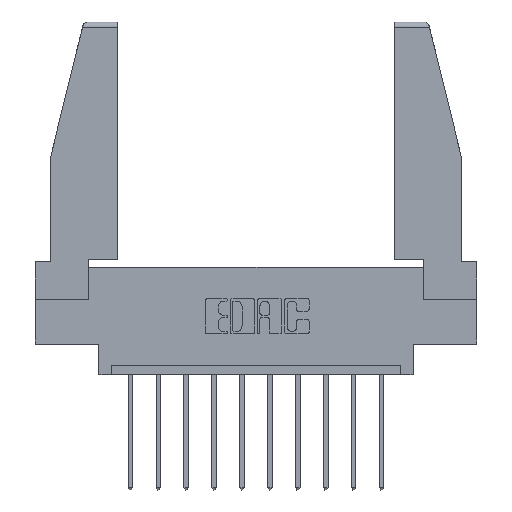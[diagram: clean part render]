
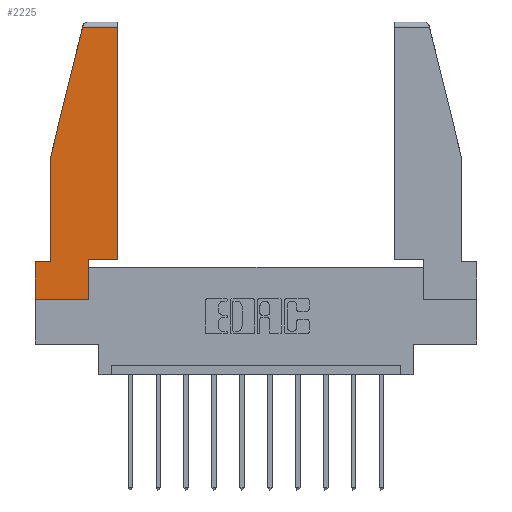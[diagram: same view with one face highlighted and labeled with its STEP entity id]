
A CAD part, top view. The second image highlights one B-rep face of the part: STEP entity #2225.
In plain terms, the highlighted planar face has unit normal (0, 0, 1).
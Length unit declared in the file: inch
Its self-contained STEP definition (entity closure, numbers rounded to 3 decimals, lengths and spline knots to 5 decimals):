
#368 = LINE ( 'NONE', #5618, #10262 ) ;
#378 = VERTEX_POINT ( 'NONE', #9417 ) ;
#496 = LINE ( 'NONE', #4893, #7648 ) ;
#766 = EDGE_CURVE ( 'NONE', #2011, #13104, #2961, .T. ) ;
#790 = CARTESIAN_POINT ( 'NONE',  ( 0.297, 0., 0. ) ) ;
#1010 = LINE ( 'NONE', #7868, #7314 ) ;
#1463 = VERTEX_POINT ( 'NONE', #4275 ) ;
#1689 = CARTESIAN_POINT ( 'NONE',  ( 0., 0., 0. ) ) ;
#1738 = CARTESIAN_POINT ( 'NONE',  ( 0.297, 0.223, 0. ) ) ;
#1741 = VECTOR ( 'NONE', #7328, 39.37008 ) ;
#1757 = CARTESIAN_POINT ( 'NONE',  ( 0., 0., 0. ) ) ;
#1901 = ORIENTED_EDGE ( 'NONE', *, *, #5869, .T. ) ;
#2002 = VERTEX_POINT ( 'NONE', #13920 ) ;
#2011 = VERTEX_POINT ( 'NONE', #790 ) ;
#2225 = ADVANCED_FACE ( 'NONE', ( #13808 ), #8231, .T. ) ;
#2400 = ORIENTED_EDGE ( 'NONE', *, *, #5689, .T. ) ;
#2610 = CARTESIAN_POINT ( 'NONE',  ( 0.2636, 1.52, 0. ) ) ;
#2647 = CARTESIAN_POINT ( 'NONE',  ( 0.271, 1.55, 0. ) ) ;
#2772 = EDGE_LOOP ( 'NONE', ( #13623, #6765, #2400, #9974, #5412, #1901, #4437, #6620, #4137 ) ) ;
#2961 = LINE ( 'NONE', #13052, #10128 ) ;
#3959 = VECTOR ( 'NONE', #10266, 39.37008 ) ;
#4137 = ORIENTED_EDGE ( 'NONE', *, *, #10483, .T. ) ;
#4158 = VECTOR ( 'NONE', #13670, 39.37008 ) ;
#4275 = CARTESIAN_POINT ( 'NONE',  ( 0.086, 0.21, 0. ) ) ;
#4437 = ORIENTED_EDGE ( 'NONE', *, *, #5126, .T. ) ;
#4545 = DIRECTION ( 'NONE',  ( 0., -1., 0. ) ) ;
#4553 = CARTESIAN_POINT ( 'NONE',  ( 0.461, 1.52, 0. ) ) ;
#4643 = LINE ( 'NONE', #7715, #5138 ) ;
#4893 = CARTESIAN_POINT ( 'NONE',  ( 0., 0.21, 0. ) ) ;
#5126 = EDGE_CURVE ( 'NONE', #2002, #2011, #12850, .T. ) ;
#5138 = VECTOR ( 'NONE', #4545, 39.37008 ) ;
#5264 = DIRECTION ( 'NONE',  ( 1., 0., 0. ) ) ;
#5412 = ORIENTED_EDGE ( 'NONE', *, *, #12501, .T. ) ;
#5604 = LINE ( 'NONE', #6216, #11063 ) ;
#5618 = CARTESIAN_POINT ( 'NONE',  ( 0., 1.52, 0. ) ) ;
#5625 = DIRECTION ( 'NONE',  ( 0., -1., 0. ) ) ;
#5689 = EDGE_CURVE ( 'NONE', #11880, #10611, #11294, .T. ) ;
#5869 = EDGE_CURVE ( 'NONE', #378, #2002, #4643, .T. ) ;
#6016 = DIRECTION ( 'NONE',  ( -1., 0., 0. ) ) ;
#6216 = CARTESIAN_POINT ( 'NONE',  ( 0.461, 0.223, 0. ) ) ;
#6609 = DIRECTION ( 'NONE',  ( -1., 0., 0. ) ) ;
#6620 = ORIENTED_EDGE ( 'NONE', *, *, #766, .T. ) ;
#6765 = ORIENTED_EDGE ( 'NONE', *, *, #10817, .T. ) ;
#7008 = LINE ( 'NONE', #13935, #1741 ) ;
#7314 = VECTOR ( 'NONE', #5625, 39.37008 ) ;
#7328 = DIRECTION ( 'NONE',  ( 1., 0., 0. ) ) ;
#7648 = VECTOR ( 'NONE', #6016, 39.37008 ) ;
#7715 = CARTESIAN_POINT ( 'NONE',  ( 0., 0.21, 0. ) ) ;
#7868 = CARTESIAN_POINT ( 'NONE',  ( 0.086, 0.8, 0. ) ) ;
#8231 = PLANE ( 'NONE',  #8969 ) ;
#8969 = AXIS2_PLACEMENT_3D ( 'NONE', #1757, #9825, #5264 ) ;
#9417 = CARTESIAN_POINT ( 'NONE',  ( 0., 0.21, 0. ) ) ;
#9654 = DIRECTION ( 'NONE',  ( 0., 1., 0. ) ) ;
#9825 = DIRECTION ( 'NONE',  ( 0., 0., 1. ) ) ;
#9974 = ORIENTED_EDGE ( 'NONE', *, *, #11491, .T. ) ;
#10128 = VECTOR ( 'NONE', #9654, 39.37008 ) ;
#10246 = VERTEX_POINT ( 'NONE', #12331 ) ;
#10262 = VECTOR ( 'NONE', #6609, 39.37008 ) ;
#10266 = DIRECTION ( 'NONE',  ( -0.239, -0.971, 0. ) ) ;
#10483 = EDGE_CURVE ( 'NONE', #13104, #10246, #7008, .T. ) ;
#10611 = VERTEX_POINT ( 'NONE', #11833 ) ;
#10622 = DIRECTION ( 'NONE',  ( 0., 1., 0. ) ) ;
#10817 = EDGE_CURVE ( 'NONE', #13071, #11880, #368, .T. ) ;
#11063 = VECTOR ( 'NONE', #10622, 39.37008 ) ;
#11294 = LINE ( 'NONE', #2647, #3959 ) ;
#11491 = EDGE_CURVE ( 'NONE', #10611, #1463, #1010, .T. ) ;
#11833 = CARTESIAN_POINT ( 'NONE',  ( 0.086, 0.8, 0. ) ) ;
#11880 = VERTEX_POINT ( 'NONE', #2610 ) ;
#12331 = CARTESIAN_POINT ( 'NONE',  ( 0.461, 0.223, 0. ) ) ;
#12501 = EDGE_CURVE ( 'NONE', #1463, #378, #496, .T. ) ;
#12783 = EDGE_CURVE ( 'NONE', #10246, #13071, #5604, .T. ) ;
#12850 = LINE ( 'NONE', #1689, #4158 ) ;
#13052 = CARTESIAN_POINT ( 'NONE',  ( 0.297, 0., 0. ) ) ;
#13071 = VERTEX_POINT ( 'NONE', #4553 ) ;
#13104 = VERTEX_POINT ( 'NONE', #1738 ) ;
#13623 = ORIENTED_EDGE ( 'NONE', *, *, #12783, .T. ) ;
#13670 = DIRECTION ( 'NONE',  ( 1., 0., 0. ) ) ;
#13808 = FACE_OUTER_BOUND ( 'NONE', #2772, .T. ) ;
#13920 = CARTESIAN_POINT ( 'NONE',  ( 0., 0., 0. ) ) ;
#13935 = CARTESIAN_POINT ( 'NONE',  ( 0.297, 0.223, 0. ) ) ;
